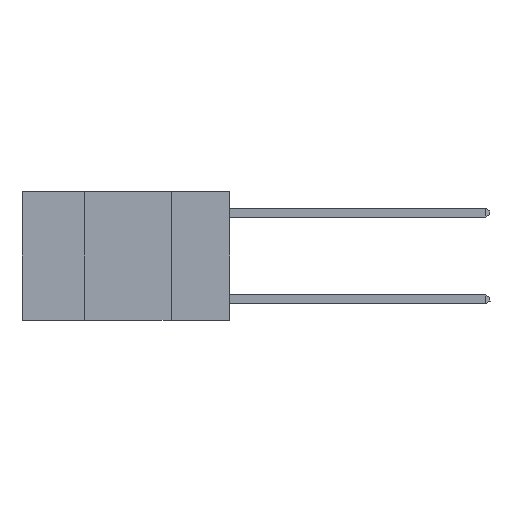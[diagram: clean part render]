
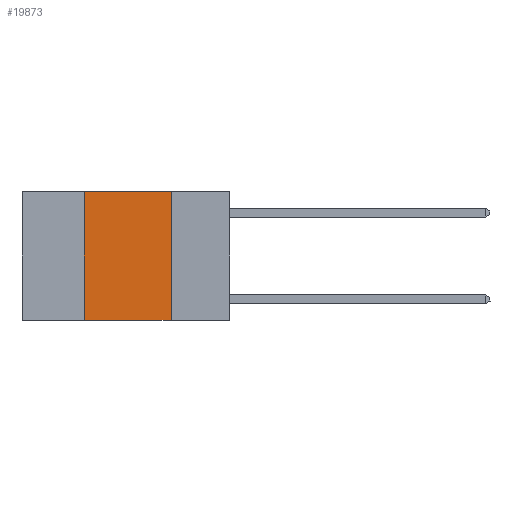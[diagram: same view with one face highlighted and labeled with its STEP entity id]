
A CAD part, left-side view. The second image highlights one B-rep face of the part: STEP entity #19873.
In plain terms, the highlighted planar face has unit normal (-1, 0, 0).
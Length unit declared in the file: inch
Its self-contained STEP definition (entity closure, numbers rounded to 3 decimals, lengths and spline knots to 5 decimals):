
#440 = LINE ( 'NONE', #21684, #16331 ) ;
#2910 = VERTEX_POINT ( 'NONE', #7901 ) ;
#3479 = EDGE_CURVE ( 'NONE', #2910, #9807, #13095, .T. ) ;
#3705 = DIRECTION ( 'NONE',  ( 0., 0., -1. ) ) ;
#3971 = CARTESIAN_POINT ( 'NONE',  ( 0., 0.42, 0. ) ) ;
#4557 = LINE ( 'NONE', #5079, #25680 ) ;
#5079 = CARTESIAN_POINT ( 'NONE',  ( 0., 0.6, -0.37 ) ) ;
#6055 = LINE ( 'NONE', #26147, #16425 ) ;
#6302 = VERTEX_POINT ( 'NONE', #6548 ) ;
#6548 = CARTESIAN_POINT ( 'NONE',  ( 0., 0.17, -0.37 ) ) ;
#7569 = VECTOR ( 'NONE', #22511, 39.37008 ) ;
#7901 = CARTESIAN_POINT ( 'NONE',  ( 0., 0.42, -0.37 ) ) ;
#8251 = CARTESIAN_POINT ( 'NONE',  ( 0., 0.6, 0. ) ) ;
#8760 = FACE_OUTER_BOUND ( 'NONE', #21730, .T. ) ;
#9504 = ORIENTED_EDGE ( 'NONE', *, *, #3479, .F. ) ;
#9807 = VERTEX_POINT ( 'NONE', #21942 ) ;
#10366 = DIRECTION ( 'NONE',  ( 0., 0., -1. ) ) ;
#12080 = AXIS2_PLACEMENT_3D ( 'NONE', #8251, #22651, #10366 ) ;
#13095 = LINE ( 'NONE', #3971, #7569 ) ;
#13460 = EDGE_CURVE ( 'NONE', #9807, #19293, #440, .T. ) ;
#14823 = CARTESIAN_POINT ( 'NONE',  ( 0., 0.17, 0. ) ) ;
#15671 = ORIENTED_EDGE ( 'NONE', *, *, #16475, .T. ) ;
#16331 = VECTOR ( 'NONE', #23671, 39.37008 ) ;
#16425 = VECTOR ( 'NONE', #3705, 39.37008 ) ;
#16475 = EDGE_CURVE ( 'NONE', #2910, #6302, #4557, .T. ) ;
#16501 = PLANE ( 'NONE',  #12080 ) ;
#19293 = VERTEX_POINT ( 'NONE', #14823 ) ;
#19873 = ADVANCED_FACE ( 'NONE', ( #8760 ), #16501, .F. ) ;
#21588 = DIRECTION ( 'NONE',  ( 0., -1., 0. ) ) ;
#21684 = CARTESIAN_POINT ( 'NONE',  ( 0., 0.6, 0. ) ) ;
#21730 = EDGE_LOOP ( 'NONE', ( #24528, #25174, #9504, #15671 ) ) ;
#21942 = CARTESIAN_POINT ( 'NONE',  ( 0., 0.42, 0. ) ) ;
#22451 = EDGE_CURVE ( 'NONE', #19293, #6302, #6055, .T. ) ;
#22511 = DIRECTION ( 'NONE',  ( 0., 0., 1. ) ) ;
#22651 = DIRECTION ( 'NONE',  ( 1., 0., 0. ) ) ;
#23671 = DIRECTION ( 'NONE',  ( 0., -1., 0. ) ) ;
#24528 = ORIENTED_EDGE ( 'NONE', *, *, #22451, .F. ) ;
#25174 = ORIENTED_EDGE ( 'NONE', *, *, #13460, .F. ) ;
#25680 = VECTOR ( 'NONE', #21588, 39.37008 ) ;
#26147 = CARTESIAN_POINT ( 'NONE',  ( 0., 0.17, 0. ) ) ;
